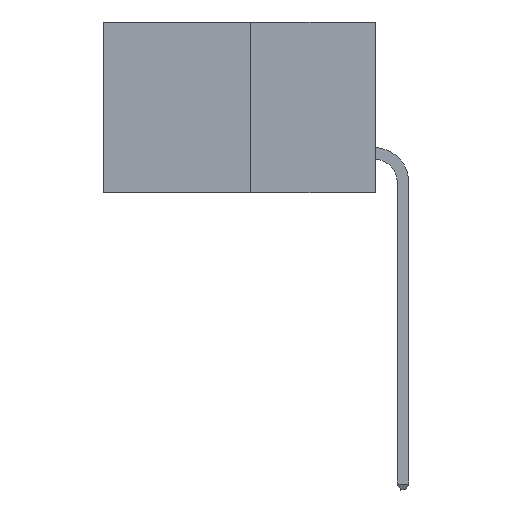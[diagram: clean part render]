
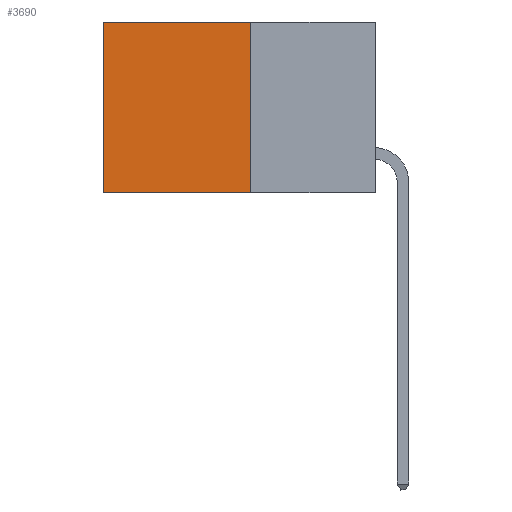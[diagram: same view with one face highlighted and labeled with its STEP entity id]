
A CAD part, left-side view. The second image highlights one B-rep face of the part: STEP entity #3690.
In plain terms, the highlighted planar face has unit normal (-1, 0, 0).
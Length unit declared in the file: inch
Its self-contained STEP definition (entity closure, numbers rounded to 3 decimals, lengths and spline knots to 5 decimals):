
#248 = VERTEX_POINT ( 'NONE', #7484 ) ;
#313 = DIRECTION ( 'NONE',  ( 0., 0., -1. ) ) ;
#475 = CARTESIAN_POINT ( 'NONE',  ( 0.277, 0.27, -0.37 ) ) ;
#540 = CARTESIAN_POINT ( 'NONE',  ( 0.277, 0.59, -0.37 ) ) ;
#950 = VECTOR ( 'NONE', #7960, 39.37008 ) ;
#1071 = LINE ( 'NONE', #8290, #3180 ) ;
#1428 = ORIENTED_EDGE ( 'NONE', *, *, #9140, .F. ) ;
#2271 = EDGE_LOOP ( 'NONE', ( #7073, #1428, #4368, #3657 ) ) ;
#2651 = PLANE ( 'NONE',  #11042 ) ;
#3180 = VECTOR ( 'NONE', #4845, 39.37008 ) ;
#3657 = ORIENTED_EDGE ( 'NONE', *, *, #10138, .T. ) ;
#3690 = ADVANCED_FACE ( 'NONE', ( #3984 ), #2651, .F. ) ;
#3984 = FACE_OUTER_BOUND ( 'NONE', #2271, .T. ) ;
#4143 = LINE ( 'NONE', #11164, #10581 ) ;
#4368 = ORIENTED_EDGE ( 'NONE', *, *, #8233, .F. ) ;
#4845 = DIRECTION ( 'NONE',  ( 0., 1., 0. ) ) ;
#5605 = LINE ( 'NONE', #7806, #950 ) ;
#6037 = CARTESIAN_POINT ( 'NONE',  ( 0.277, 0.59, -0.37 ) ) ;
#7073 = ORIENTED_EDGE ( 'NONE', *, *, #9025, .T. ) ;
#7286 = VECTOR ( 'NONE', #313, 39.37008 ) ;
#7473 = CARTESIAN_POINT ( 'NONE',  ( 0.277, 0.27, -0.37 ) ) ;
#7484 = CARTESIAN_POINT ( 'NONE',  ( 0.277, 0.27, 0. ) ) ;
#7514 = VERTEX_POINT ( 'NONE', #6037 ) ;
#7806 = CARTESIAN_POINT ( 'NONE',  ( 0.277, 0.27, -0.37 ) ) ;
#7960 = DIRECTION ( 'NONE',  ( 0., 0., -1. ) ) ;
#8233 = EDGE_CURVE ( 'NONE', #248, #8252, #5605, .T. ) ;
#8252 = VERTEX_POINT ( 'NONE', #7473 ) ;
#8290 = CARTESIAN_POINT ( 'NONE',  ( 0.277, 0.27, 0. ) ) ;
#9025 = EDGE_CURVE ( 'NONE', #9087, #7514, #9538, .T. ) ;
#9087 = VERTEX_POINT ( 'NONE', #9777 ) ;
#9140 = EDGE_CURVE ( 'NONE', #8252, #7514, #4143, .T. ) ;
#9538 = LINE ( 'NONE', #540, #7286 ) ;
#9777 = CARTESIAN_POINT ( 'NONE',  ( 0.277, 0.59, 0. ) ) ;
#10028 = DIRECTION ( 'NONE',  ( 1., 0., 0. ) ) ;
#10057 = DIRECTION ( 'NONE',  ( 0., 0., -1. ) ) ;
#10138 = EDGE_CURVE ( 'NONE', #248, #9087, #1071, .T. ) ;
#10468 = DIRECTION ( 'NONE',  ( 0., 1., 0. ) ) ;
#10581 = VECTOR ( 'NONE', #10468, 39.37008 ) ;
#11042 = AXIS2_PLACEMENT_3D ( 'NONE', #475, #10028, #10057 ) ;
#11164 = CARTESIAN_POINT ( 'NONE',  ( 0.277, 0.27, -0.37 ) ) ;
